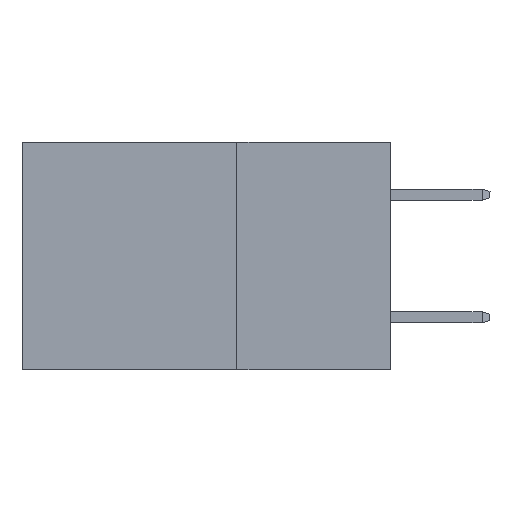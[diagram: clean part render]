
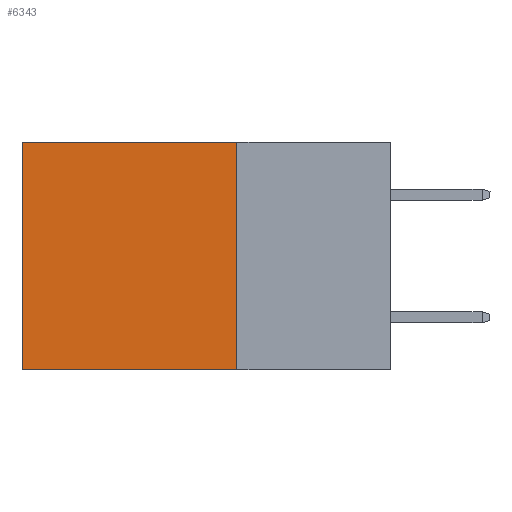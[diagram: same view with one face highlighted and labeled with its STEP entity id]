
A CAD part, left-side view. The second image highlights one B-rep face of the part: STEP entity #6343.
In plain terms, the highlighted planar face has unit normal (-1, 0, 0).
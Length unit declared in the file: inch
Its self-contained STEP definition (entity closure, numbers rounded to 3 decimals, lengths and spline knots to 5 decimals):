
#68 = VECTOR ( 'NONE', #3098, 39.37008 ) ;
#416 = VECTOR ( 'NONE', #11002, 39.37008 ) ;
#905 = CARTESIAN_POINT ( 'NONE',  ( 0.2875, 0.25, -0.37 ) ) ;
#1112 = VECTOR ( 'NONE', #1839, 39.37008 ) ;
#1808 = VECTOR ( 'NONE', #2098, 39.37008 ) ;
#1839 = DIRECTION ( 'NONE',  ( 0., 1., 0. ) ) ;
#2098 = DIRECTION ( 'NONE',  ( 0., 0., -1. ) ) ;
#2106 = CARTESIAN_POINT ( 'NONE',  ( 0.2875, 0.25, -0.37 ) ) ;
#2244 = ORIENTED_EDGE ( 'NONE', *, *, #14407, .F. ) ;
#2462 = VERTEX_POINT ( 'NONE', #7356 ) ;
#3038 = EDGE_CURVE ( 'NONE', #2462, #13711, #14567, .T. ) ;
#3098 = DIRECTION ( 'NONE',  ( 0., 0., -1. ) ) ;
#3326 = AXIS2_PLACEMENT_3D ( 'NONE', #13150, #14282, #7082 ) ;
#3539 = LINE ( 'NONE', #13059, #68 ) ;
#3714 = EDGE_LOOP ( 'NONE', ( #4785, #13506, #2244, #12795 ) ) ;
#4130 = CARTESIAN_POINT ( 'NONE',  ( 0.2875, 0.25, 0. ) ) ;
#4571 = LINE ( 'NONE', #13096, #1112 ) ;
#4785 = ORIENTED_EDGE ( 'NONE', *, *, #3038, .T. ) ;
#4963 = FACE_OUTER_BOUND ( 'NONE', #3714, .T. ) ;
#6312 = EDGE_CURVE ( 'NONE', #7479, #2462, #4571, .T. ) ;
#6343 = ADVANCED_FACE ( 'NONE', ( #4963 ), #11929, .F. ) ;
#7082 = DIRECTION ( 'NONE',  ( 0., 0., -1. ) ) ;
#7356 = CARTESIAN_POINT ( 'NONE',  ( 0.2875, 0.6, 0. ) ) ;
#7479 = VERTEX_POINT ( 'NONE', #4130 ) ;
#10247 = LINE ( 'NONE', #2106, #416 ) ;
#10602 = EDGE_CURVE ( 'NONE', #11760, #13711, #10247, .T. ) ;
#11002 = DIRECTION ( 'NONE',  ( 0., 1., 0. ) ) ;
#11760 = VERTEX_POINT ( 'NONE', #905 ) ;
#11929 = PLANE ( 'NONE',  #3326 ) ;
#12795 = ORIENTED_EDGE ( 'NONE', *, *, #6312, .T. ) ;
#13059 = CARTESIAN_POINT ( 'NONE',  ( 0.2875, 0.25, 0. ) ) ;
#13096 = CARTESIAN_POINT ( 'NONE',  ( 0.2875, 0.25, 0. ) ) ;
#13150 = CARTESIAN_POINT ( 'NONE',  ( 0.2875, 0.25, 0. ) ) ;
#13506 = ORIENTED_EDGE ( 'NONE', *, *, #10602, .F. ) ;
#13614 = CARTESIAN_POINT ( 'NONE',  ( 0.2875, 0.6, -0.37 ) ) ;
#13711 = VERTEX_POINT ( 'NONE', #13614 ) ;
#14282 = DIRECTION ( 'NONE',  ( 1., 0., 0. ) ) ;
#14407 = EDGE_CURVE ( 'NONE', #7479, #11760, #3539, .T. ) ;
#14415 = CARTESIAN_POINT ( 'NONE',  ( 0.2875, 0.6, 0. ) ) ;
#14567 = LINE ( 'NONE', #14415, #1808 ) ;
